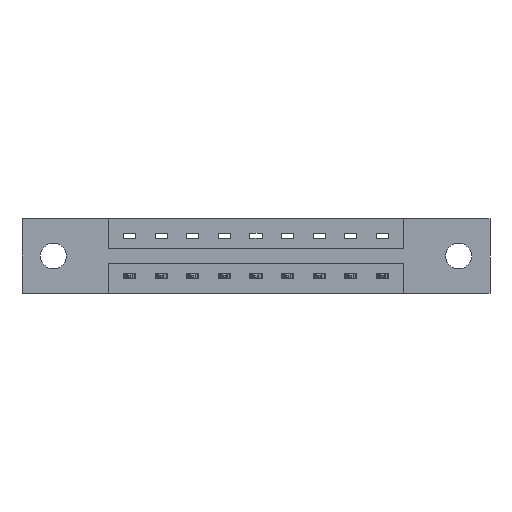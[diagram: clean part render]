
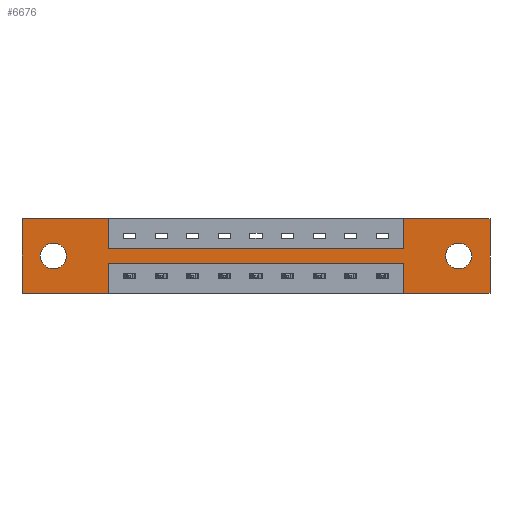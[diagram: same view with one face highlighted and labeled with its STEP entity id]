
A CAD part, front view. The second image highlights one B-rep face of the part: STEP entity #6676.
In plain terms, the highlighted planar face has unit normal (0, -1, 0).
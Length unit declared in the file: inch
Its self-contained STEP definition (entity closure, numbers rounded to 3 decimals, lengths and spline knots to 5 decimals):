
#67 = VERTEX_POINT ( 'NONE', #7985 ) ;
#119 = LINE ( 'NONE', #306, #5553 ) ;
#128 = CARTESIAN_POINT ( 'NONE',  ( 0.425, 0., -0.22 ) ) ;
#217 = CARTESIAN_POINT ( 'NONE',  ( 0.425, 0., -0.37 ) ) ;
#291 = CARTESIAN_POINT ( 'NONE',  ( 0.425, 0., 0. ) ) ;
#306 = CARTESIAN_POINT ( 'NONE',  ( 1.885, 0., -0.37 ) ) ;
#387 = CARTESIAN_POINT ( 'NONE',  ( 1.885, 0., -0.22 ) ) ;
#399 = CARTESIAN_POINT ( 'NONE',  ( 0., 0., 0. ) ) ;
#408 = ORIENTED_EDGE ( 'NONE', *, *, #5954, .F. ) ;
#547 = DIRECTION ( 'NONE',  ( 1., 0., 0. ) ) ;
#553 = ORIENTED_EDGE ( 'NONE', *, *, #6764, .F. ) ;
#580 = LINE ( 'NONE', #3009, #10403 ) ;
#581 = DIRECTION ( 'NONE',  ( 0., 0., -1. ) ) ;
#841 = ORIENTED_EDGE ( 'NONE', *, *, #6876, .T. ) ;
#843 = VERTEX_POINT ( 'NONE', #5300 ) ;
#1098 = DIRECTION ( 'NONE',  ( 0., 1., 0. ) ) ;
#1148 = AXIS2_PLACEMENT_3D ( 'NONE', #3656, #1098, #10394 ) ;
#1221 = VERTEX_POINT ( 'NONE', #8153 ) ;
#1228 = DIRECTION ( 'NONE',  ( 0., 0., 1. ) ) ;
#1380 = EDGE_CURVE ( 'NONE', #8898, #4910, #5352, .T. ) ;
#1418 = VERTEX_POINT ( 'NONE', #217 ) ;
#1485 = CARTESIAN_POINT ( 'NONE',  ( 0., 0., -0.37 ) ) ;
#1506 = EDGE_CURVE ( 'NONE', #843, #67, #1873, .T. ) ;
#1670 = CARTESIAN_POINT ( 'NONE',  ( 0.155, 0., -0.249 ) ) ;
#1707 = LINE ( 'NONE', #6425, #10740 ) ;
#1873 = LINE ( 'NONE', #291, #8138 ) ;
#1982 = CARTESIAN_POINT ( 'NONE',  ( 0., 0., 0. ) ) ;
#2052 = VECTOR ( 'NONE', #3527, 39.37008 ) ;
#2183 = VERTEX_POINT ( 'NONE', #9483 ) ;
#2187 = EDGE_LOOP ( 'NONE', ( #5255, #841 ) ) ;
#2197 = DIRECTION ( 'NONE',  ( 1., 0., 0. ) ) ;
#2255 = DIRECTION ( 'NONE',  ( 0., -1., 0. ) ) ;
#2300 = FACE_BOUND ( 'NONE', #2187, .T. ) ;
#2400 = LINE ( 'NONE', #2561, #6651 ) ;
#2448 = CARTESIAN_POINT ( 'NONE',  ( 2.31, 0., -0.37 ) ) ;
#2512 = EDGE_CURVE ( 'NONE', #67, #9199, #1707, .T. ) ;
#2561 = CARTESIAN_POINT ( 'NONE',  ( 0.425, 0., -0.37 ) ) ;
#2837 = DIRECTION ( 'NONE',  ( 0., 1., 0. ) ) ;
#2853 = CIRCLE ( 'NONE', #6877, 0.064 ) ;
#2897 = ORIENTED_EDGE ( 'NONE', *, *, #1380, .F. ) ;
#3009 = CARTESIAN_POINT ( 'NONE',  ( 0., 0., 0. ) ) ;
#3227 = LINE ( 'NONE', #128, #3497 ) ;
#3303 = DIRECTION ( 'NONE',  ( 0., 1., 0. ) ) ;
#3364 = VECTOR ( 'NONE', #1228, 39.37008 ) ;
#3497 = VECTOR ( 'NONE', #9434, 39.37008 ) ;
#3514 = VECTOR ( 'NONE', #6237, 39.37008 ) ;
#3527 = DIRECTION ( 'NONE',  ( 0., 0., 1. ) ) ;
#3656 = CARTESIAN_POINT ( 'NONE',  ( 0.155, 0., -0.185 ) ) ;
#3778 = ORIENTED_EDGE ( 'NONE', *, *, #6219, .F. ) ;
#3918 = VECTOR ( 'NONE', #9704, 39.37008 ) ;
#3920 = CARTESIAN_POINT ( 'NONE',  ( 2.31, 0., 0. ) ) ;
#3936 = ORIENTED_EDGE ( 'NONE', *, *, #8943, .F. ) ;
#4370 = ORIENTED_EDGE ( 'NONE', *, *, #10911, .F. ) ;
#4387 = EDGE_CURVE ( 'NONE', #9199, #7787, #5677, .T. ) ;
#4441 = ORIENTED_EDGE ( 'NONE', *, *, #6170, .F. ) ;
#4561 = CIRCLE ( 'NONE', #9002, 0.064 ) ;
#4827 = EDGE_CURVE ( 'NONE', #1221, #10563, #4998, .T. ) ;
#4828 = FACE_OUTER_BOUND ( 'NONE', #7636, .T. ) ;
#4910 = VERTEX_POINT ( 'NONE', #399 ) ;
#4959 = CARTESIAN_POINT ( 'NONE',  ( 0.155, 0., -0.185 ) ) ;
#4998 = CIRCLE ( 'NONE', #1148, 0.064 ) ;
#5017 = CARTESIAN_POINT ( 'NONE',  ( 1.885, 0., 0. ) ) ;
#5255 = ORIENTED_EDGE ( 'NONE', *, *, #4827, .T. ) ;
#5300 = CARTESIAN_POINT ( 'NONE',  ( 0.425, 0., 0. ) ) ;
#5352 = LINE ( 'NONE', #1982, #3364 ) ;
#5355 = CARTESIAN_POINT ( 'NONE',  ( 0., 0., 0. ) ) ;
#5372 = AXIS2_PLACEMENT_3D ( 'NONE', #10704, #2255, #581 ) ;
#5455 = EDGE_LOOP ( 'NONE', ( #8483, #7323 ) ) ;
#5553 = VECTOR ( 'NONE', #6244, 39.37008 ) ;
#5564 = PLANE ( 'NONE',  #5372 ) ;
#5677 = LINE ( 'NONE', #10150, #2052 ) ;
#5851 = CARTESIAN_POINT ( 'NONE',  ( 0.425, 0., -0.22 ) ) ;
#5862 = DIRECTION ( 'NONE',  ( 0., 1., 0. ) ) ;
#5873 = LINE ( 'NONE', #9162, #10503 ) ;
#5954 = EDGE_CURVE ( 'NONE', #7214, #9710, #7000, .T. ) ;
#5967 = ORIENTED_EDGE ( 'NONE', *, *, #9770, .F. ) ;
#6170 = EDGE_CURVE ( 'NONE', #4910, #843, #9615, .T. ) ;
#6181 = DIRECTION ( 'NONE',  ( 0., 0., -1. ) ) ;
#6219 = EDGE_CURVE ( 'NONE', #7787, #7214, #580, .T. ) ;
#6237 = DIRECTION ( 'NONE',  ( -1., 0., 0. ) ) ;
#6244 = DIRECTION ( 'NONE',  ( 0., 0., 1. ) ) ;
#6373 = EDGE_CURVE ( 'NONE', #2183, #8886, #2853, .T. ) ;
#6425 = CARTESIAN_POINT ( 'NONE',  ( 0.425, 0., -0.15 ) ) ;
#6651 = VECTOR ( 'NONE', #9320, 39.37008 ) ;
#6676 = ADVANCED_FACE ( 'NONE', ( #8031, #2300, #4828 ), #5564, .T. ) ;
#6764 = EDGE_CURVE ( 'NONE', #1418, #8898, #7647, .T. ) ;
#6835 = CIRCLE ( 'NONE', #8988, 0.064 ) ;
#6876 = EDGE_CURVE ( 'NONE', #10563, #1221, #6835, .T. ) ;
#6877 = AXIS2_PLACEMENT_3D ( 'NONE', #10441, #2837, #8774 ) ;
#6997 = CARTESIAN_POINT ( 'NONE',  ( 0., 0., -0.37 ) ) ;
#7000 = LINE ( 'NONE', #3920, #7137 ) ;
#7137 = VECTOR ( 'NONE', #6181, 39.37008 ) ;
#7214 = VERTEX_POINT ( 'NONE', #10348 ) ;
#7323 = ORIENTED_EDGE ( 'NONE', *, *, #6373, .T. ) ;
#7562 = CARTESIAN_POINT ( 'NONE',  ( 2.155, 0., -0.185 ) ) ;
#7636 = EDGE_LOOP ( 'NONE', ( #5967, #3936, #4370, #7717, #408, #3778, #10575, #9141, #10341, #4441, #2897, #553 ) ) ;
#7647 = LINE ( 'NONE', #6997, #3514 ) ;
#7717 = ORIENTED_EDGE ( 'NONE', *, *, #8701, .F. ) ;
#7787 = VERTEX_POINT ( 'NONE', #5017 ) ;
#7985 = CARTESIAN_POINT ( 'NONE',  ( 0.425, 0., -0.15 ) ) ;
#8031 = FACE_BOUND ( 'NONE', #5455, .T. ) ;
#8138 = VECTOR ( 'NONE', #10423, 39.37008 ) ;
#8153 = CARTESIAN_POINT ( 'NONE',  ( 0.155, 0., -0.121 ) ) ;
#8316 = DIRECTION ( 'NONE',  ( -1., 0., 0. ) ) ;
#8483 = ORIENTED_EDGE ( 'NONE', *, *, #8583, .T. ) ;
#8583 = EDGE_CURVE ( 'NONE', #8886, #2183, #4561, .T. ) ;
#8599 = CARTESIAN_POINT ( 'NONE',  ( 1.885, 0., -0.15 ) ) ;
#8701 = EDGE_CURVE ( 'NONE', #9710, #10410, #5873, .T. ) ;
#8774 = DIRECTION ( 'NONE',  ( 0., 0., -1. ) ) ;
#8886 = VERTEX_POINT ( 'NONE', #10691 ) ;
#8898 = VERTEX_POINT ( 'NONE', #1485 ) ;
#8943 = EDGE_CURVE ( 'NONE', #10749, #10496, #3227, .T. ) ;
#8988 = AXIS2_PLACEMENT_3D ( 'NONE', #4959, #3303, #9218 ) ;
#9002 = AXIS2_PLACEMENT_3D ( 'NONE', #7562, #5862, #9387 ) ;
#9041 = CARTESIAN_POINT ( 'NONE',  ( 1.885, 0., -0.37 ) ) ;
#9141 = ORIENTED_EDGE ( 'NONE', *, *, #2512, .F. ) ;
#9162 = CARTESIAN_POINT ( 'NONE',  ( 0., 0., -0.37 ) ) ;
#9199 = VERTEX_POINT ( 'NONE', #8599 ) ;
#9218 = DIRECTION ( 'NONE',  ( 0., 0., 1. ) ) ;
#9320 = DIRECTION ( 'NONE',  ( 0., 0., -1. ) ) ;
#9387 = DIRECTION ( 'NONE',  ( 0., 0., -1. ) ) ;
#9434 = DIRECTION ( 'NONE',  ( -1., 0., 0. ) ) ;
#9483 = CARTESIAN_POINT ( 'NONE',  ( 2.155, 0., -0.249 ) ) ;
#9615 = LINE ( 'NONE', #5355, #3918 ) ;
#9704 = DIRECTION ( 'NONE',  ( 1., 0., 0. ) ) ;
#9710 = VERTEX_POINT ( 'NONE', #2448 ) ;
#9770 = EDGE_CURVE ( 'NONE', #10496, #1418, #2400, .T. ) ;
#10150 = CARTESIAN_POINT ( 'NONE',  ( 1.885, 0., 0. ) ) ;
#10341 = ORIENTED_EDGE ( 'NONE', *, *, #1506, .F. ) ;
#10348 = CARTESIAN_POINT ( 'NONE',  ( 2.31, 0., 0. ) ) ;
#10394 = DIRECTION ( 'NONE',  ( 0., 0., 1. ) ) ;
#10403 = VECTOR ( 'NONE', #2197, 39.37008 ) ;
#10410 = VERTEX_POINT ( 'NONE', #9041 ) ;
#10423 = DIRECTION ( 'NONE',  ( 0., 0., -1. ) ) ;
#10441 = CARTESIAN_POINT ( 'NONE',  ( 2.155, 0., -0.185 ) ) ;
#10496 = VERTEX_POINT ( 'NONE', #5851 ) ;
#10503 = VECTOR ( 'NONE', #8316, 39.37008 ) ;
#10563 = VERTEX_POINT ( 'NONE', #1670 ) ;
#10575 = ORIENTED_EDGE ( 'NONE', *, *, #4387, .F. ) ;
#10691 = CARTESIAN_POINT ( 'NONE',  ( 2.155, 0., -0.121 ) ) ;
#10704 = CARTESIAN_POINT ( 'NONE',  ( 0., 0., -0.37 ) ) ;
#10740 = VECTOR ( 'NONE', #547, 39.37008 ) ;
#10749 = VERTEX_POINT ( 'NONE', #387 ) ;
#10911 = EDGE_CURVE ( 'NONE', #10410, #10749, #119, .T. ) ;
